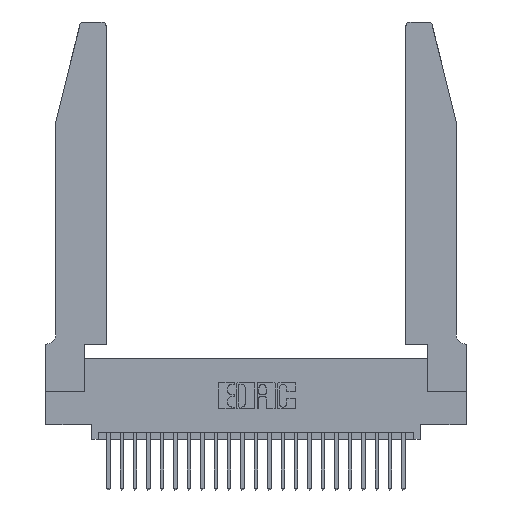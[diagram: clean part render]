
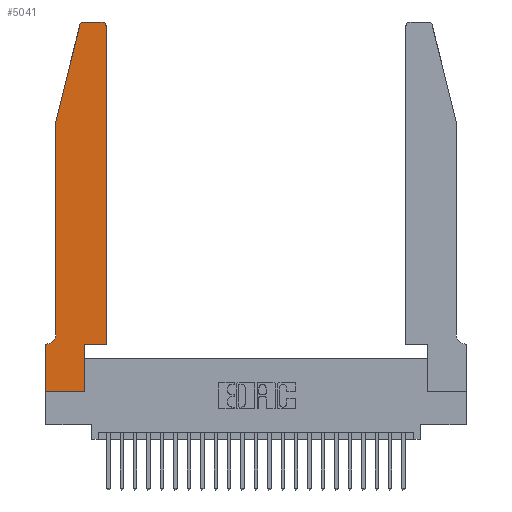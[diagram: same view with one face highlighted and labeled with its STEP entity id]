
A CAD part, top view. The second image highlights one B-rep face of the part: STEP entity #5041.
In plain terms, the highlighted planar face has unit normal (0, 0, 1).
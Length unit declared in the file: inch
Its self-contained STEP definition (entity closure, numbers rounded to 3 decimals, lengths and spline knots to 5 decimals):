
#19 = ORIENTED_EDGE ( 'NONE', *, *, #9540, .T. ) ;
#271 = CARTESIAN_POINT ( 'NONE',  ( 0.284, 2.72, 0.37 ) ) ;
#477 = VERTEX_POINT ( 'NONE', #19748 ) ;
#540 = EDGE_CURVE ( 'NONE', #13186, #9649, #4530, .T. ) ;
#643 = DIRECTION ( 'NONE',  ( -1., 0., 0. ) ) ;
#909 = VECTOR ( 'NONE', #15488, 39.37008 ) ;
#973 = CARTESIAN_POINT ( 'NONE',  ( 0.0755, 0.42, 0.37 ) ) ;
#1017 = CARTESIAN_POINT ( 'NONE',  ( 0.4505, 2.72, 0.37 ) ) ;
#1121 = ORIENTED_EDGE ( 'NONE', *, *, #21939, .T. ) ;
#1438 = CARTESIAN_POINT ( 'NONE',  ( 0.2865, 0., 0.37 ) ) ;
#1815 = DIRECTION ( 'NONE',  ( 1., 0., 0. ) ) ;
#1841 = LINE ( 'NONE', #11284, #18238 ) ;
#1957 = CARTESIAN_POINT ( 'NONE',  ( 0.4205, 2.72, 0.37 ) ) ;
#2330 = ORIENTED_EDGE ( 'NONE', *, *, #3699, .T. ) ;
#2585 = FACE_OUTER_BOUND ( 'NONE', #22305, .T. ) ;
#2595 = DIRECTION ( 'NONE',  ( 0., -1., 0. ) ) ;
#2667 = LINE ( 'NONE', #19019, #16288 ) ;
#2869 = VECTOR ( 'NONE', #24643, 39.37008 ) ;
#2953 = LINE ( 'NONE', #14126, #17223 ) ;
#3212 = CARTESIAN_POINT ( 'NONE',  ( 0., 0., 0.37 ) ) ;
#3586 = EDGE_CURVE ( 'NONE', #9994, #5800, #6041, .T. ) ;
#3699 = EDGE_CURVE ( 'NONE', #15431, #6083, #2953, .T. ) ;
#4157 = VERTEX_POINT ( 'NONE', #24188 ) ;
#4530 = LINE ( 'NONE', #12201, #24283 ) ;
#5041 = ADVANCED_FACE ( 'NONE', ( #2585 ), #13819, .T. ) ;
#5800 = VERTEX_POINT ( 'NONE', #17421 ) ;
#5841 = CARTESIAN_POINT ( 'NONE',  ( 0., 0.35, 0.37 ) ) ;
#6041 = CIRCLE ( 'NONE', #7134, 0.03 ) ;
#6083 = VERTEX_POINT ( 'NONE', #18706 ) ;
#6187 = LINE ( 'NONE', #9694, #909 ) ;
#6346 = DIRECTION ( 'NONE',  ( 0., 1., 0. ) ) ;
#6895 = CARTESIAN_POINT ( 'NONE',  ( 0.4505, 0.35, 0.37 ) ) ;
#7001 = ORIENTED_EDGE ( 'NONE', *, *, #20615, .T. ) ;
#7134 = AXIS2_PLACEMENT_3D ( 'NONE', #1957, #9920, #21569 ) ;
#7340 = VECTOR ( 'NONE', #2595, 39.37008 ) ;
#7704 = DIRECTION ( 'NONE',  ( 0., 0., 1. ) ) ;
#7846 = LINE ( 'NONE', #6895, #2869 ) ;
#8035 = ORIENTED_EDGE ( 'NONE', *, *, #18648, .T. ) ;
#9540 = EDGE_CURVE ( 'NONE', #10877, #15431, #6187, .T. ) ;
#9649 = VERTEX_POINT ( 'NONE', #24798 ) ;
#9694 = CARTESIAN_POINT ( 'NONE',  ( 0., 0., 0.37 ) ) ;
#9920 = DIRECTION ( 'NONE',  ( 0., 0., 1. ) ) ;
#9994 = VERTEX_POINT ( 'NONE', #1017 ) ;
#10069 = DIRECTION ( 'NONE',  ( -0.239, -0.971, 0. ) ) ;
#10346 = VECTOR ( 'NONE', #22988, 39.37008 ) ;
#10589 = VECTOR ( 'NONE', #19453, 39.37008 ) ;
#10877 = VERTEX_POINT ( 'NONE', #12975 ) ;
#11284 = CARTESIAN_POINT ( 'NONE',  ( 0.2605, 2.75, 0.37 ) ) ;
#12201 = CARTESIAN_POINT ( 'NONE',  ( 0.0755, 2., 0.37 ) ) ;
#12476 = ORIENTED_EDGE ( 'NONE', *, *, #15780, .T. ) ;
#12494 = DIRECTION ( 'NONE',  ( 0., 0., -1. ) ) ;
#12516 = ORIENTED_EDGE ( 'NONE', *, *, #21424, .T. ) ;
#12523 = DIRECTION ( 'NONE',  ( 1., 0., 0. ) ) ;
#12975 = CARTESIAN_POINT ( 'NONE',  ( 0., 0., 0.37 ) ) ;
#13186 = VERTEX_POINT ( 'NONE', #18419 ) ;
#13819 = PLANE ( 'NONE',  #16324 ) ;
#14014 = CARTESIAN_POINT ( 'NONE',  ( 0.284, 2.75, 0.37 ) ) ;
#14126 = CARTESIAN_POINT ( 'NONE',  ( 0.2865, 0.35, 0.37 ) ) ;
#14657 = EDGE_CURVE ( 'NONE', #9649, #21746, #22774, .T. ) ;
#15300 = DIRECTION ( 'NONE',  ( -1., 0., 0. ) ) ;
#15309 = LINE ( 'NONE', #3212, #10346 ) ;
#15431 = VERTEX_POINT ( 'NONE', #1438 ) ;
#15488 = DIRECTION ( 'NONE',  ( 1., 0., 0. ) ) ;
#15780 = EDGE_CURVE ( 'NONE', #23831, #13186, #17195, .T. ) ;
#15940 = ORIENTED_EDGE ( 'NONE', *, *, #20818, .T. ) ;
#16288 = VECTOR ( 'NONE', #15300, 39.37008 ) ;
#16324 = AXIS2_PLACEMENT_3D ( 'NONE', #21587, #7704, #1815 ) ;
#16873 = CIRCLE ( 'NONE', #25282, 0.07 ) ;
#17195 = CIRCLE ( 'NONE', #21283, 0.03 ) ;
#17223 = VECTOR ( 'NONE', #6346, 39.37008 ) ;
#17347 = EDGE_CURVE ( 'NONE', #6083, #4157, #21690, .T. ) ;
#17421 = CARTESIAN_POINT ( 'NONE',  ( 0.4205, 2.75, 0.37 ) ) ;
#17521 = ORIENTED_EDGE ( 'NONE', *, *, #3586, .T. ) ;
#18204 = ORIENTED_EDGE ( 'NONE', *, *, #14657, .T. ) ;
#18238 = VECTOR ( 'NONE', #24767, 39.37008 ) ;
#18419 = CARTESIAN_POINT ( 'NONE',  ( 0.25487, 2.72718, 0.37 ) ) ;
#18648 = EDGE_CURVE ( 'NONE', #5800, #23831, #1841, .T. ) ;
#18706 = CARTESIAN_POINT ( 'NONE',  ( 0.2865, 0.35, 0.37 ) ) ;
#19019 = CARTESIAN_POINT ( 'NONE',  ( 0.0755, 0.35, 0.37 ) ) ;
#19066 = ORIENTED_EDGE ( 'NONE', *, *, #17347, .T. ) ;
#19453 = DIRECTION ( 'NONE',  ( 1., 0., 0. ) ) ;
#19748 = CARTESIAN_POINT ( 'NONE',  ( 0.0055, 0.35, 0.37 ) ) ;
#19795 = ORIENTED_EDGE ( 'NONE', *, *, #540, .T. ) ;
#20363 = CARTESIAN_POINT ( 'NONE',  ( 0.0055, 0.42, 0.37 ) ) ;
#20615 = EDGE_CURVE ( 'NONE', #477, #20744, #2667, .T. ) ;
#20744 = VERTEX_POINT ( 'NONE', #5841 ) ;
#20818 = EDGE_CURVE ( 'NONE', #21746, #477, #16873, .T. ) ;
#21283 = AXIS2_PLACEMENT_3D ( 'NONE', #271, #22374, #12523 ) ;
#21424 = EDGE_CURVE ( 'NONE', #20744, #10877, #15309, .T. ) ;
#21569 = DIRECTION ( 'NONE',  ( 1., 0., 0. ) ) ;
#21587 = CARTESIAN_POINT ( 'NONE',  ( 0., 0.35, 0.37 ) ) ;
#21687 = CARTESIAN_POINT ( 'NONE',  ( 0.4505, 0.35, 0.37 ) ) ;
#21690 = LINE ( 'NONE', #21687, #10589 ) ;
#21746 = VERTEX_POINT ( 'NONE', #973 ) ;
#21939 = EDGE_CURVE ( 'NONE', #4157, #9994, #7846, .T. ) ;
#22305 = EDGE_LOOP ( 'NONE', ( #8035, #12476, #19795, #18204, #15940, #7001, #12516, #19, #2330, #19066, #1121, #17521 ) ) ;
#22374 = DIRECTION ( 'NONE',  ( 0., 0., 1. ) ) ;
#22774 = LINE ( 'NONE', #24225, #7340 ) ;
#22988 = DIRECTION ( 'NONE',  ( 0., -1., 0. ) ) ;
#23831 = VERTEX_POINT ( 'NONE', #14014 ) ;
#24188 = CARTESIAN_POINT ( 'NONE',  ( 0.4505, 0.35, 0.37 ) ) ;
#24225 = CARTESIAN_POINT ( 'NONE',  ( 0.0755, 2., 0.37 ) ) ;
#24283 = VECTOR ( 'NONE', #10069, 39.37008 ) ;
#24643 = DIRECTION ( 'NONE',  ( 0., 1., 0. ) ) ;
#24767 = DIRECTION ( 'NONE',  ( -1., 0., 0. ) ) ;
#24798 = CARTESIAN_POINT ( 'NONE',  ( 0.0755, 2., 0.37 ) ) ;
#25282 = AXIS2_PLACEMENT_3D ( 'NONE', #20363, #12494, #643 ) ;
